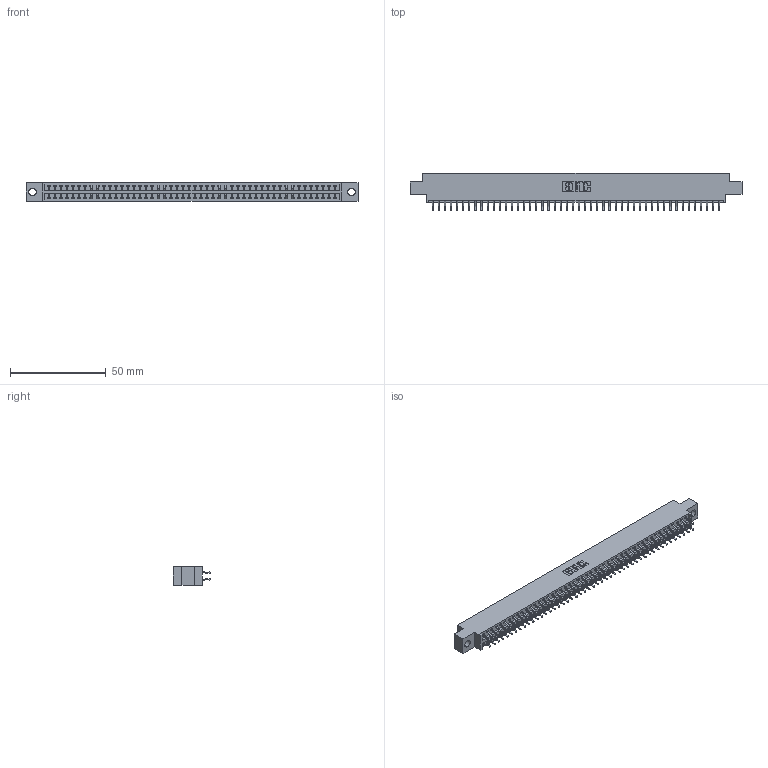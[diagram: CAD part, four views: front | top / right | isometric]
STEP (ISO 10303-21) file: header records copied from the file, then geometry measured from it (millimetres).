
FILE_DESCRIPTION (( 'STEP AP203' ), '1' );
FILE_NAME ('396-096-556-804.STEP', '2019-11-02T16:50:18', ( '' ), ( '' ), 'SwSTEP 2.0', 'SolidWorks 2016', '' );
FILE_SCHEMA (( 'CONFIG_CONTROL_DESIGN' ));
Length unit declared in the file: inch
Products named in the file (3): 346 Part_0.170 Offset - 0.156 Dia-TH; 345-292-001_556 Tail; 396-096-556-804
Assembly tree (97 placements, depth 2):
  396-096-556-804
    346 Part_0.170 Offset - 0.156 Dia-TH
    345-292-001_556 Tail  x96
Bounding box: 172.97 x 19.57 x 9.4 mm (x, y, z)
Volume: 16667.4 mm3; surface area: 22908.6 mm2
Topology: 97 solids, 97 shells, 5694 faces, 16949 edges, 11170 vertices
Faces by surface type: plane 3824, cylinder 1870
Entity records: 30873 total; most frequent: CARTESIAN_POINT 5096, ORIENTED_EDGE 5018, DIRECTION 4529, EDGE_CURVE 2509, LINE 2177, VECTOR 2177, VERTEX_POINT 1670, AXIS2_PLACEMENT_3D 1176
